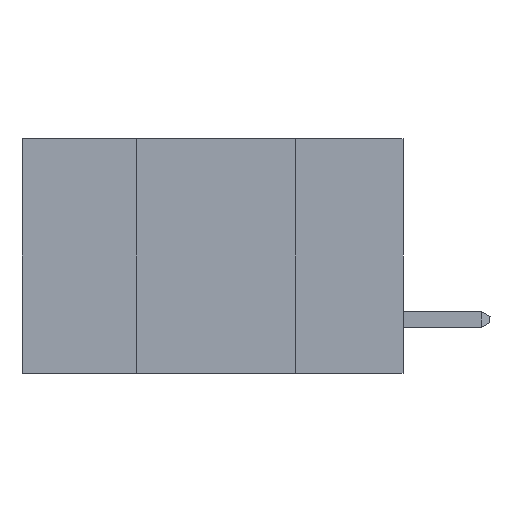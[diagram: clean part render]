
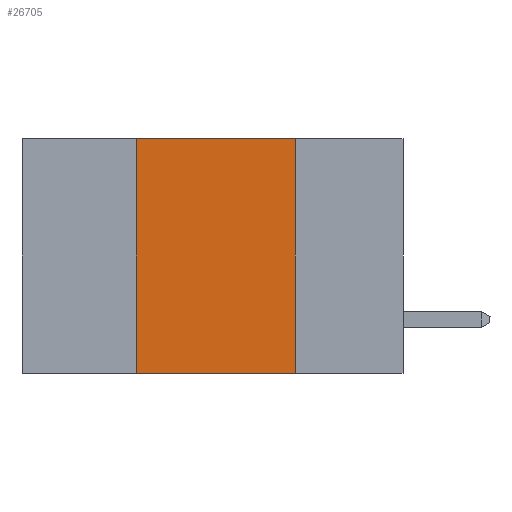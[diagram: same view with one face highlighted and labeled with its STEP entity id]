
A CAD part, left-side view. The second image highlights one B-rep face of the part: STEP entity #26705.
In plain terms, the highlighted planar face has unit normal (-1, 0, 0).
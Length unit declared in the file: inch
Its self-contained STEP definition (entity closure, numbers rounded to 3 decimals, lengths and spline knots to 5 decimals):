
#871 = VECTOR ( 'NONE', #1147, 39.37008 ) ;
#1147 = DIRECTION ( 'NONE',  ( 0., -1., 0. ) ) ;
#1286 = LINE ( 'NONE', #29165, #33628 ) ;
#1872 = DIRECTION ( 'NONE',  ( 0., -1., 0. ) ) ;
#2201 = DIRECTION ( 'NONE',  ( 0., 0., -1. ) ) ;
#4757 = VERTEX_POINT ( 'NONE', #11427 ) ;
#6085 = CARTESIAN_POINT ( 'NONE',  ( 0., 0.6, 0. ) ) ;
#8602 = CARTESIAN_POINT ( 'NONE',  ( 0., 0.17, 0. ) ) ;
#11427 = CARTESIAN_POINT ( 'NONE',  ( 0., 0.42, -0.37 ) ) ;
#11676 = EDGE_CURVE ( 'NONE', #12973, #24962, #1286, .T. ) ;
#11712 = CARTESIAN_POINT ( 'NONE',  ( 0., 0.6, 0. ) ) ;
#12973 = VERTEX_POINT ( 'NONE', #8602 ) ;
#13349 = VECTOR ( 'NONE', #37604, 39.37008 ) ;
#13812 = EDGE_LOOP ( 'NONE', ( #18985, #44528, #17395, #34204 ) ) ;
#14219 = EDGE_CURVE ( 'NONE', #4757, #24962, #32457, .T. ) ;
#16385 = DIRECTION ( 'NONE',  ( 1., 0., 0. ) ) ;
#17395 = ORIENTED_EDGE ( 'NONE', *, *, #37627, .F. ) ;
#18985 = ORIENTED_EDGE ( 'NONE', *, *, #11676, .F. ) ;
#23621 = VECTOR ( 'NONE', #1872, 39.37008 ) ;
#24962 = VERTEX_POINT ( 'NONE', #29466 ) ;
#25370 = CARTESIAN_POINT ( 'NONE',  ( 0., 0.6, -0.37 ) ) ;
#26308 = LINE ( 'NONE', #11712, #23621 ) ;
#26705 = ADVANCED_FACE ( 'NONE', ( #37149 ), #30999, .F. ) ;
#29165 = CARTESIAN_POINT ( 'NONE',  ( 0., 0.17, 0. ) ) ;
#29213 = EDGE_CURVE ( 'NONE', #38763, #12973, #26308, .T. ) ;
#29291 = AXIS2_PLACEMENT_3D ( 'NONE', #6085, #16385, #2201 ) ;
#29466 = CARTESIAN_POINT ( 'NONE',  ( 0., 0.17, -0.37 ) ) ;
#30067 = CARTESIAN_POINT ( 'NONE',  ( 0., 0.42, 0. ) ) ;
#30999 = PLANE ( 'NONE',  #29291 ) ;
#31097 = CARTESIAN_POINT ( 'NONE',  ( 0., 0.42, 0. ) ) ;
#32457 = LINE ( 'NONE', #25370, #871 ) ;
#33628 = VECTOR ( 'NONE', #43096, 39.37008 ) ;
#34204 = ORIENTED_EDGE ( 'NONE', *, *, #14219, .T. ) ;
#37149 = FACE_OUTER_BOUND ( 'NONE', #13812, .T. ) ;
#37604 = DIRECTION ( 'NONE',  ( 0., 0., 1. ) ) ;
#37627 = EDGE_CURVE ( 'NONE', #4757, #38763, #40791, .T. ) ;
#38763 = VERTEX_POINT ( 'NONE', #31097 ) ;
#40791 = LINE ( 'NONE', #30067, #13349 ) ;
#43096 = DIRECTION ( 'NONE',  ( 0., 0., -1. ) ) ;
#44528 = ORIENTED_EDGE ( 'NONE', *, *, #29213, .F. ) ;
